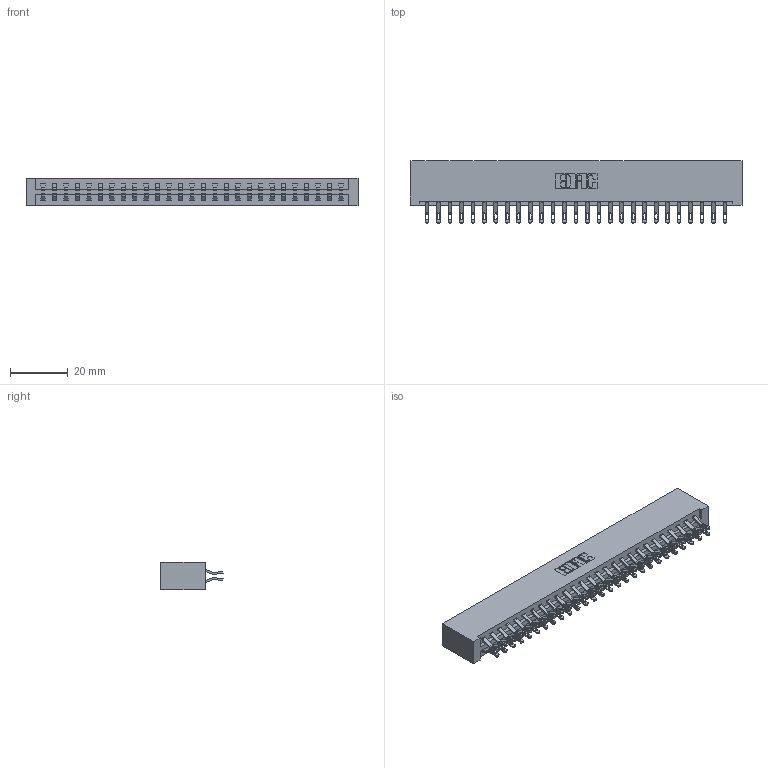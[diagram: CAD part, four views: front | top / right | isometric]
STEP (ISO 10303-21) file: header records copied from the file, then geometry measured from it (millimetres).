
FILE_DESCRIPTION (( 'STEP AP203' ), '1' );
FILE_NAME ('337-054-555-201.STEP', '2019-10-09T18:14:47', ( '' ), ( '' ), 'SwSTEP 2.0', 'SolidWorks 2016', '' );
FILE_SCHEMA (( 'CONFIG_CONTROL_DESIGN' ));
Length unit declared in the file: inch
Products named in the file (3): 337 Part_No Mounting Lugs; 337-054-555-201; 345-292-001_555 Tail
Assembly tree (55 placements, depth 2):
  337-054-555-201
    337 Part_No Mounting Lugs
    345-292-001_555 Tail  x54
Bounding box: 114.86 x 21.47 x 9.4 mm (x, y, z)
Volume: 12822.4 mm3; surface area: 14996.4 mm2
Topology: 55 solids, 55 shells, 3346 faces, 10493 edges, 6994 vertices
Faces by surface type: plane 2010, cylinder 1336
Entity records: 22923 total; most frequent: CARTESIAN_POINT 3908, ORIENTED_EDGE 3814, DIRECTION 3315, EDGE_CURVE 1907, VECTOR 1767, LINE 1767, VERTEX_POINT 1270, AXIS2_PLACEMENT_3D 774
